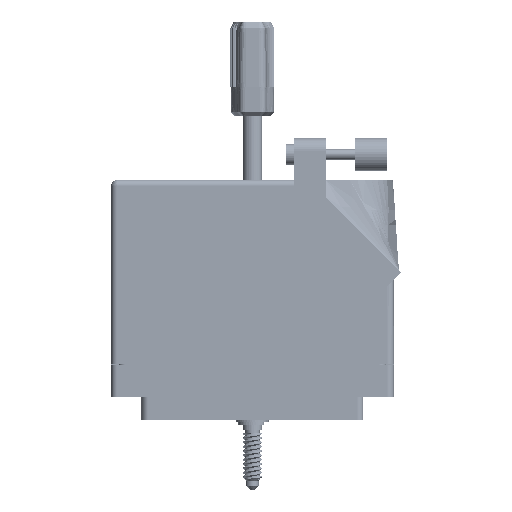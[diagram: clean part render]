
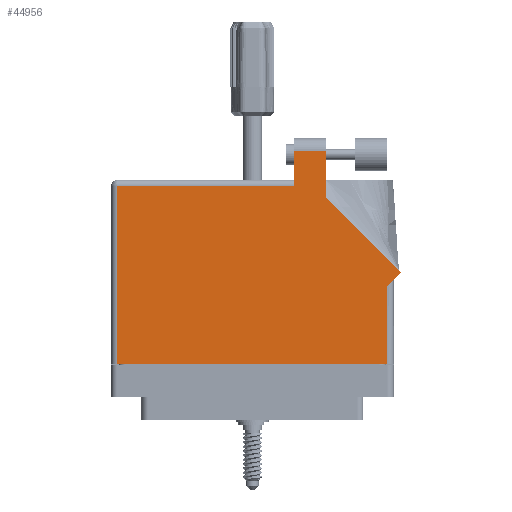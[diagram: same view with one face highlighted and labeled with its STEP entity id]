
A CAD part, front view. The second image highlights one B-rep face of the part: STEP entity #44956.
In plain terms, the highlighted face is planar.
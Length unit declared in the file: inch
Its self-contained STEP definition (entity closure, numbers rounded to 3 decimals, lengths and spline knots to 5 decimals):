
#70 = EDGE_CURVE ( 'NONE', #26850, #27597, #43285, .T. ) ;
#1044 = VECTOR ( 'NONE', #84487, 39.37008 ) ;
#3266 = EDGE_CURVE ( 'NONE', #36514, #27822, #17711, .T. ) ;
#8931 = CARTESIAN_POINT ( 'NONE',  ( 1.359, 0.715, 0.617 ) ) ;
#11197 = DIRECTION ( 'NONE',  ( 0., 0., -1. ) ) ;
#12585 = EDGE_CURVE ( 'NONE', #86160, #49022, #52031, .T. ) ;
#13339 = EDGE_CURVE ( 'NONE', #73378, #86160, #17701, .T. ) ;
#14295 = VERTEX_POINT ( 'NONE', #16120 ) ;
#15681 = DIRECTION ( 'NONE',  ( 0.707, 0.707, 0. ) ) ;
#16120 = CARTESIAN_POINT ( 'NONE',  ( 0.399, 1.95, 0.617 ) ) ;
#17701 = LINE ( 'NONE', #71601, #1044 ) ;
#17711 = LINE ( 'NONE', #67544, #62954 ) ;
#17899 = PLANE ( 'NONE',  #50343 ) ;
#22280 = CARTESIAN_POINT ( 'NONE',  ( 0.399, 1.613, 0.617 ) ) ;
#24271 = EDGE_CURVE ( 'NONE', #14295, #26850, #53301, .T. ) ;
#25406 = CARTESIAN_POINT ( 'NONE',  ( -1.297, -0.1, 0.617 ) ) ;
#25854 = FACE_OUTER_BOUND ( 'NONE', #65524, .T. ) ;
#26850 = VERTEX_POINT ( 'NONE', #22280 ) ;
#27597 = VERTEX_POINT ( 'NONE', #32197 ) ;
#27822 = VERTEX_POINT ( 'NONE', #48281 ) ;
#29508 = ORIENTED_EDGE ( 'NONE', *, *, #3266, .T. ) ;
#30241 = CARTESIAN_POINT ( 'NONE',  ( 0.399, 1.95, 0.617 ) ) ;
#31705 = EDGE_CURVE ( 'NONE', #49022, #14295, #72132, .T. ) ;
#32197 = CARTESIAN_POINT ( 'NONE',  ( -1.297, 1.613, 0.617 ) ) ;
#34260 = ORIENTED_EDGE ( 'NONE', *, *, #13339, .T. ) ;
#34498 = CARTESIAN_POINT ( 'NONE',  ( 0.399, 1.675, 0.617 ) ) ;
#35396 = VECTOR ( 'NONE', #67127, 39.37008 ) ;
#35517 = CARTESIAN_POINT ( 'NONE',  ( -1.297, -0.1, 0.617 ) ) ;
#36227 = VECTOR ( 'NONE', #63976, 39.37008 ) ;
#36514 = VERTEX_POINT ( 'NONE', #56284 ) ;
#37848 = DIRECTION ( 'NONE',  ( -1., 0., 0. ) ) ;
#38366 = VECTOR ( 'NONE', #44761, 39.37008 ) ;
#39436 = EDGE_CURVE ( 'NONE', #27822, #73378, #70910, .T. ) ;
#39832 = EDGE_CURVE ( 'NONE', #27597, #78089, #47739, .T. ) ;
#40450 = ORIENTED_EDGE ( 'NONE', *, *, #39832, .T. ) ;
#41454 = VECTOR ( 'NONE', #68156, 39.37008 ) ;
#43285 = LINE ( 'NONE', #66358, #63329 ) ;
#43935 = CARTESIAN_POINT ( 'NONE',  ( -1.359, -0.1, 0.617 ) ) ;
#44761 = DIRECTION ( 'NONE',  ( 0., 1., 0. ) ) ;
#44956 = ADVANCED_FACE ( 'NONE', ( #25854 ), #17899, .F. ) ;
#46589 = DIRECTION ( 'NONE',  ( -1., 0., 0. ) ) ;
#47739 = LINE ( 'NONE', #35517, #41454 ) ;
#48281 = CARTESIAN_POINT ( 'NONE',  ( 1.297, 0.653, 0.617 ) ) ;
#49022 = VERTEX_POINT ( 'NONE', #59476 ) ;
#50015 = ORIENTED_EDGE ( 'NONE', *, *, #39436, .T. ) ;
#50343 = AXIS2_PLACEMENT_3D ( 'NONE', #78021, #11197, #58162 ) ;
#51853 = CARTESIAN_POINT ( 'NONE',  ( 0.706, 1.50942, 0.617 ) ) ;
#52031 = LINE ( 'NONE', #51853, #38366 ) ;
#53301 = LINE ( 'NONE', #34498, #35396 ) ;
#56284 = CARTESIAN_POINT ( 'NONE',  ( 1.297, -0.1, 0.617 ) ) ;
#58162 = DIRECTION ( 'NONE',  ( -1., 0., 0. ) ) ;
#58345 = LINE ( 'NONE', #43935, #36227 ) ;
#59476 = CARTESIAN_POINT ( 'NONE',  ( 0.706, 1.95, 0.617 ) ) ;
#59648 = ORIENTED_EDGE ( 'NONE', *, *, #60095, .T. ) ;
#60095 = EDGE_CURVE ( 'NONE', #78089, #36514, #58345, .T. ) ;
#60472 = VECTOR ( 'NONE', #15681, 39.37008 ) ;
#60880 = CARTESIAN_POINT ( 'NONE',  ( 0.706, 1.50942, 0.617 ) ) ;
#62954 = VECTOR ( 'NONE', #80676, 39.37008 ) ;
#63329 = VECTOR ( 'NONE', #46589, 39.37008 ) ;
#63747 = VECTOR ( 'NONE', #37848, 39.37008 ) ;
#63976 = DIRECTION ( 'NONE',  ( 1., 0., 0. ) ) ;
#64040 = ORIENTED_EDGE ( 'NONE', *, *, #24271, .T. ) ;
#65524 = EDGE_LOOP ( 'NONE', ( #73917, #71576, #64040, #81357, #40450, #59648, #29508, #50015, #34260 ) ) ;
#66358 = CARTESIAN_POINT ( 'NONE',  ( -1.359, 1.613, 0.617 ) ) ;
#67018 = CARTESIAN_POINT ( 'NONE',  ( 1.42971, 0.78571, 0.617 ) ) ;
#67127 = DIRECTION ( 'NONE',  ( 0., -1., 0. ) ) ;
#67544 = CARTESIAN_POINT ( 'NONE',  ( 1.297, 0.715, 0.617 ) ) ;
#68156 = DIRECTION ( 'NONE',  ( 0., -1., 0. ) ) ;
#70910 = LINE ( 'NONE', #8931, #60472 ) ;
#71576 = ORIENTED_EDGE ( 'NONE', *, *, #31705, .T. ) ;
#71601 = CARTESIAN_POINT ( 'NONE',  ( 1.42971, 0.78571, 0.617 ) ) ;
#72132 = LINE ( 'NONE', #30241, #63747 ) ;
#73378 = VERTEX_POINT ( 'NONE', #67018 ) ;
#73917 = ORIENTED_EDGE ( 'NONE', *, *, #12585, .T. ) ;
#78021 = CARTESIAN_POINT ( 'NONE',  ( -1.359, 1.675, 0.617 ) ) ;
#78089 = VERTEX_POINT ( 'NONE', #25406 ) ;
#80676 = DIRECTION ( 'NONE',  ( 0., 1., 0. ) ) ;
#81357 = ORIENTED_EDGE ( 'NONE', *, *, #70, .T. ) ;
#84487 = DIRECTION ( 'NONE',  ( -0.707, 0.707, 0. ) ) ;
#86160 = VERTEX_POINT ( 'NONE', #60880 ) ;
